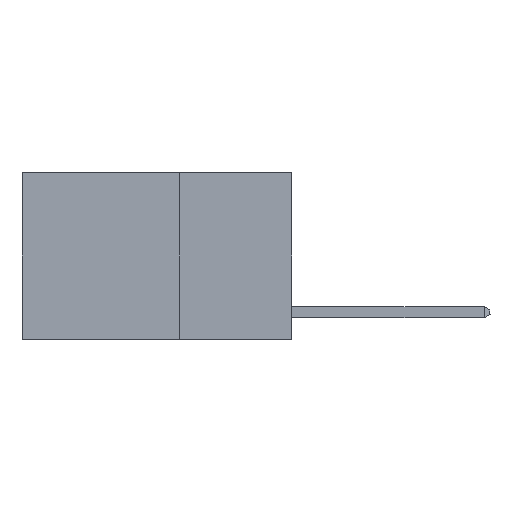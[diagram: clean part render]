
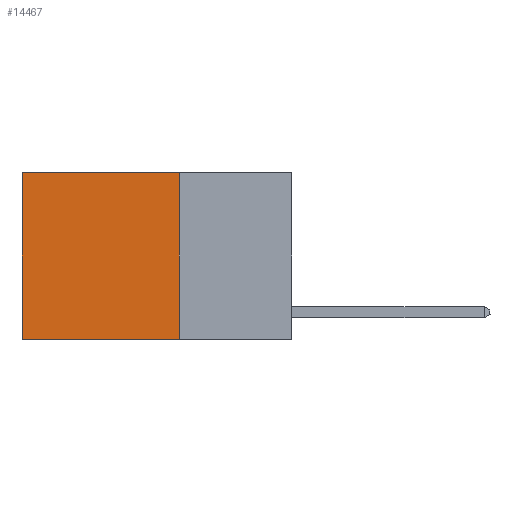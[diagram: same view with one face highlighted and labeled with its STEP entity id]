
A CAD part, left-side view. The second image highlights one B-rep face of the part: STEP entity #14467.
In plain terms, the highlighted planar face has unit normal (-1, 0, 0).
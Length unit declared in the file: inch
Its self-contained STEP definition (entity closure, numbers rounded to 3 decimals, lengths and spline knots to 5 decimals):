
#4 = ORIENTED_EDGE ( 'NONE', *, *, #7796, .F. ) ;
#195 = EDGE_CURVE ( 'NONE', #9300, #13040, #3949, .T. ) ;
#1108 = ORIENTED_EDGE ( 'NONE', *, *, #5110, .F. ) ;
#2108 = DIRECTION ( 'NONE',  ( 0., 0., -1. ) ) ;
#2260 = PLANE ( 'NONE',  #10444 ) ;
#3035 = CARTESIAN_POINT ( 'NONE',  ( 0.2625, 0.6, 0. ) ) ;
#3949 = LINE ( 'NONE', #9981, #8609 ) ;
#4631 = VECTOR ( 'NONE', #6394, 39.37008 ) ;
#5110 = EDGE_CURVE ( 'NONE', #9300, #11388, #15199, .T. ) ;
#5131 = CARTESIAN_POINT ( 'NONE',  ( 0.2625, 0.25, 0. ) ) ;
#5904 = CARTESIAN_POINT ( 'NONE',  ( 0.2625, 0.25, 0. ) ) ;
#6394 = DIRECTION ( 'NONE',  ( 0., 1., 0. ) ) ;
#7796 = EDGE_CURVE ( 'NONE', #11388, #15228, #11182, .T. ) ;
#8192 = ORIENTED_EDGE ( 'NONE', *, *, #12456, .T. ) ;
#8375 = ORIENTED_EDGE ( 'NONE', *, *, #195, .T. ) ;
#8448 = DIRECTION ( 'NONE',  ( 0., 1., 0. ) ) ;
#8609 = VECTOR ( 'NONE', #8448, 39.37008 ) ;
#9046 = CARTESIAN_POINT ( 'NONE',  ( 0.2625, 0.6, 0. ) ) ;
#9061 = DIRECTION ( 'NONE',  ( 0., 0., -1. ) ) ;
#9300 = VERTEX_POINT ( 'NONE', #5131 ) ;
#9981 = CARTESIAN_POINT ( 'NONE',  ( 0.2625, 0.25, 0. ) ) ;
#10318 = CARTESIAN_POINT ( 'NONE',  ( 0.2625, 0.25, 0. ) ) ;
#10362 = LINE ( 'NONE', #3035, #14148 ) ;
#10444 = AXIS2_PLACEMENT_3D ( 'NONE', #5904, #11622, #10619 ) ;
#10619 = DIRECTION ( 'NONE',  ( 0., 0., -1. ) ) ;
#11182 = LINE ( 'NONE', #13601, #4631 ) ;
#11269 = CARTESIAN_POINT ( 'NONE',  ( 0.2625, 0.6, -0.37 ) ) ;
#11388 = VERTEX_POINT ( 'NONE', #15236 ) ;
#11622 = DIRECTION ( 'NONE',  ( 1., 0., 0. ) ) ;
#11865 = VECTOR ( 'NONE', #2108, 39.37008 ) ;
#12456 = EDGE_CURVE ( 'NONE', #13040, #15228, #10362, .T. ) ;
#12844 = EDGE_LOOP ( 'NONE', ( #8192, #4, #1108, #8375 ) ) ;
#13040 = VERTEX_POINT ( 'NONE', #9046 ) ;
#13601 = CARTESIAN_POINT ( 'NONE',  ( 0.2625, 0.25, -0.37 ) ) ;
#14111 = FACE_OUTER_BOUND ( 'NONE', #12844, .T. ) ;
#14148 = VECTOR ( 'NONE', #9061, 39.37008 ) ;
#14467 = ADVANCED_FACE ( 'NONE', ( #14111 ), #2260, .F. ) ;
#15199 = LINE ( 'NONE', #10318, #11865 ) ;
#15228 = VERTEX_POINT ( 'NONE', #11269 ) ;
#15236 = CARTESIAN_POINT ( 'NONE',  ( 0.2625, 0.25, -0.37 ) ) ;
